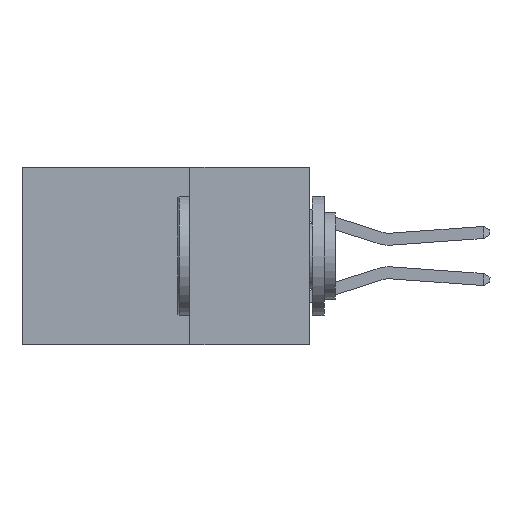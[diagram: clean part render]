
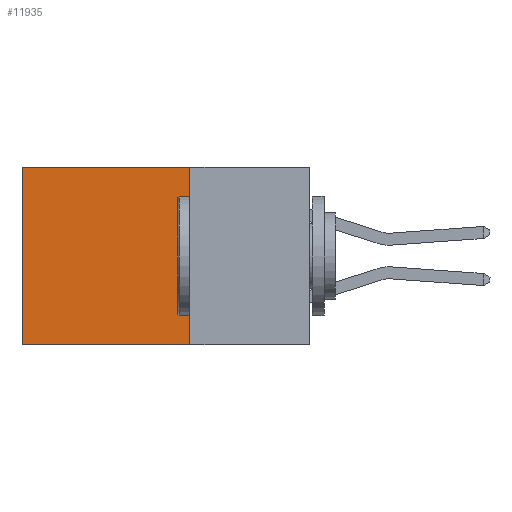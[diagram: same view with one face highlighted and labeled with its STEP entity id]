
A CAD part, left-side view. The second image highlights one B-rep face of the part: STEP entity #11935.
In plain terms, the highlighted planar face has unit normal (-1, 0, 0).
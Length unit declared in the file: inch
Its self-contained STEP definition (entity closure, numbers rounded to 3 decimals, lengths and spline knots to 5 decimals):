
#276 = CARTESIAN_POINT ( 'NONE',  ( 0.2615, 0.6, 0. ) ) ;
#730 = LINE ( 'NONE', #10660, #12055 ) ;
#1255 = VERTEX_POINT ( 'NONE', #18127 ) ;
#1344 = EDGE_CURVE ( 'NONE', #11059, #13285, #4553, .T. ) ;
#2128 = ORIENTED_EDGE ( 'NONE', *, *, #21038, .T. ) ;
#2937 = PLANE ( 'NONE',  #20281 ) ;
#4357 = DIRECTION ( 'NONE',  ( 0., 0., -1. ) ) ;
#4553 = LINE ( 'NONE', #8417, #9909 ) ;
#4849 = CARTESIAN_POINT ( 'NONE',  ( 0.2615, 0.25, -0.37 ) ) ;
#4938 = DIRECTION ( 'NONE',  ( 1., 0., 0. ) ) ;
#4991 = CARTESIAN_POINT ( 'NONE',  ( 0.2615, 0.25, 0. ) ) ;
#6250 = LINE ( 'NONE', #12518, #16344 ) ;
#6543 = VECTOR ( 'NONE', #17064, 39.37008 ) ;
#8417 = CARTESIAN_POINT ( 'NONE',  ( 0.2615, 0.6, -0.37 ) ) ;
#9561 = ORIENTED_EDGE ( 'NONE', *, *, #1344, .T. ) ;
#9909 = VECTOR ( 'NONE', #4357, 39.37008 ) ;
#10660 = CARTESIAN_POINT ( 'NONE',  ( 0.2615, 0.25, -0.37 ) ) ;
#10962 = ORIENTED_EDGE ( 'NONE', *, *, #15255, .F. ) ;
#11059 = VERTEX_POINT ( 'NONE', #276 ) ;
#11935 = ADVANCED_FACE ( 'NONE', ( #14093 ), #2937, .F. ) ;
#12055 = VECTOR ( 'NONE', #12712, 39.37008 ) ;
#12518 = CARTESIAN_POINT ( 'NONE',  ( 0.2615, 0.25, -0.37 ) ) ;
#12712 = DIRECTION ( 'NONE',  ( 0., 0., -1. ) ) ;
#13245 = CARTESIAN_POINT ( 'NONE',  ( 0.2615, 0.25, -0.37 ) ) ;
#13285 = VERTEX_POINT ( 'NONE', #24318 ) ;
#14093 = FACE_OUTER_BOUND ( 'NONE', #14540, .T. ) ;
#14540 = EDGE_LOOP ( 'NONE', ( #9561, #21600, #10962, #2128 ) ) ;
#15255 = EDGE_CURVE ( 'NONE', #1255, #15400, #730, .T. ) ;
#15400 = VERTEX_POINT ( 'NONE', #13245 ) ;
#16010 = LINE ( 'NONE', #4991, #6543 ) ;
#16344 = VECTOR ( 'NONE', #18526, 39.37008 ) ;
#17064 = DIRECTION ( 'NONE',  ( 0., 1., 0. ) ) ;
#17076 = EDGE_CURVE ( 'NONE', #15400, #13285, #6250, .T. ) ;
#18127 = CARTESIAN_POINT ( 'NONE',  ( 0.2615, 0.25, 0. ) ) ;
#18526 = DIRECTION ( 'NONE',  ( 0., 1., 0. ) ) ;
#19062 = DIRECTION ( 'NONE',  ( 0., 0., -1. ) ) ;
#20281 = AXIS2_PLACEMENT_3D ( 'NONE', #4849, #4938, #19062 ) ;
#21038 = EDGE_CURVE ( 'NONE', #1255, #11059, #16010, .T. ) ;
#21600 = ORIENTED_EDGE ( 'NONE', *, *, #17076, .F. ) ;
#24318 = CARTESIAN_POINT ( 'NONE',  ( 0.2615, 0.6, -0.37 ) ) ;
